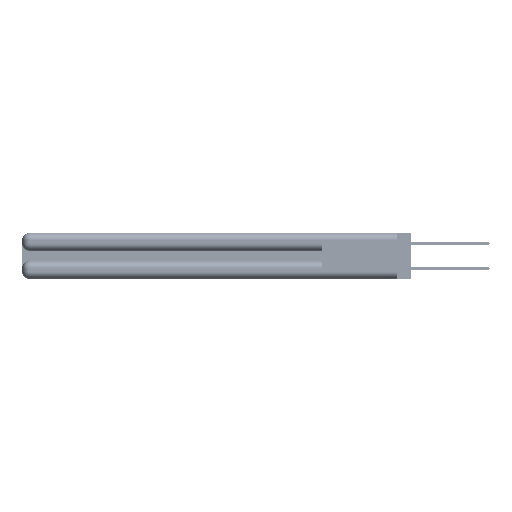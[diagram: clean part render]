
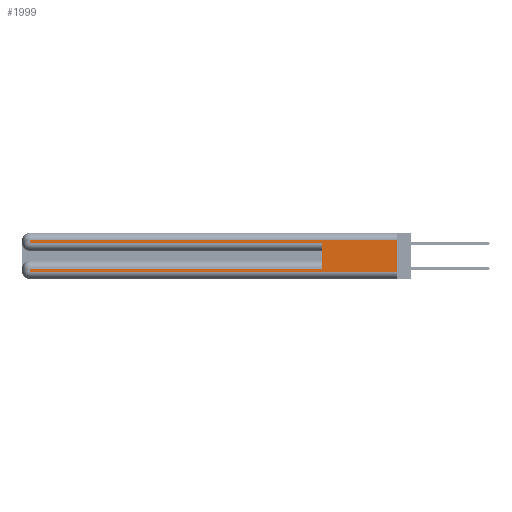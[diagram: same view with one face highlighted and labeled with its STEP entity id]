
A CAD part, left-side view. The second image highlights one B-rep face of the part: STEP entity #1999.
In plain terms, the highlighted planar face has unit normal (-1, 0, 0).
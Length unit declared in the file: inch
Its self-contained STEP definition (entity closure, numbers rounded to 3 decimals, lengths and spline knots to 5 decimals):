
#1750 = FACE_OUTER_BOUND ( 'NONE', #46465, .T. ) ;
#1999 = ADVANCED_FACE ( 'NONE', ( #1750 ), #5914, .F. ) ;
#3607 = ORIENTED_EDGE ( 'NONE', *, *, #37052, .T. ) ;
#3769 = ORIENTED_EDGE ( 'NONE', *, *, #54869, .T. ) ;
#4452 = DIRECTION ( 'NONE',  ( 0., 0., -1. ) ) ;
#4638 = CARTESIAN_POINT ( 'NONE',  ( 0., 2.94, 0.37 ) ) ;
#5604 = LINE ( 'NONE', #4638, #40401 ) ;
#5707 = LINE ( 'NONE', #15758, #15888 ) ;
#5914 = PLANE ( 'NONE',  #20199 ) ;
#6242 = VECTOR ( 'NONE', #30039, 39.37008 ) ;
#8123 = CARTESIAN_POINT ( 'NONE',  ( 0., 0.6, 0.085 ) ) ;
#9010 = DIRECTION ( 'NONE',  ( 0., 0., -1. ) ) ;
#10978 = CARTESIAN_POINT ( 'NONE',  ( 0., 0., 0.085 ) ) ;
#10979 = VECTOR ( 'NONE', #9010, 39.37008 ) ;
#12269 = CARTESIAN_POINT ( 'NONE',  ( 0., 0., 0.31 ) ) ;
#13804 = VECTOR ( 'NONE', #45222, 39.37008 ) ;
#14412 = VERTEX_POINT ( 'NONE', #39367 ) ;
#14622 = DIRECTION ( 'NONE',  ( 0., 0., -1. ) ) ;
#15758 = CARTESIAN_POINT ( 'NONE',  ( 0., 0., 0.37 ) ) ;
#15888 = VECTOR ( 'NONE', #20144, 39.37008 ) ;
#16745 = ORIENTED_EDGE ( 'NONE', *, *, #27738, .F. ) ;
#17822 = LINE ( 'NONE', #25661, #6242 ) ;
#20144 = DIRECTION ( 'NONE',  ( 0., 0., -1. ) ) ;
#20199 = AXIS2_PLACEMENT_3D ( 'NONE', #36408, #40789, #14622 ) ;
#24513 = VERTEX_POINT ( 'NONE', #43925 ) ;
#24615 = ORIENTED_EDGE ( 'NONE', *, *, #28487, .T. ) ;
#24803 = VERTEX_POINT ( 'NONE', #41235 ) ;
#25661 = CARTESIAN_POINT ( 'NONE',  ( 0., 0., 0.06 ) ) ;
#27361 = DIRECTION ( 'NONE',  ( 0., -1., 0. ) ) ;
#27738 = EDGE_CURVE ( 'NONE', #33438, #24513, #5707, .T. ) ;
#28165 = LINE ( 'NONE', #41052, #13804 ) ;
#28487 = EDGE_CURVE ( 'NONE', #36521, #36227, #44465, .T. ) ;
#30039 = DIRECTION ( 'NONE',  ( 0., -1., 0. ) ) ;
#31236 = VERTEX_POINT ( 'NONE', #44261 ) ;
#31534 = VECTOR ( 'NONE', #37148, 39.37008 ) ;
#32031 = VECTOR ( 'NONE', #27361, 39.37008 ) ;
#32733 = CARTESIAN_POINT ( 'NONE',  ( 0., 0.6, 0.145 ) ) ;
#33438 = VERTEX_POINT ( 'NONE', #12269 ) ;
#35183 = CARTESIAN_POINT ( 'NONE',  ( 0., 2.94, 0.37 ) ) ;
#36227 = VERTEX_POINT ( 'NONE', #48456 ) ;
#36408 = CARTESIAN_POINT ( 'NONE',  ( 0., 0., 0.37 ) ) ;
#36521 = VERTEX_POINT ( 'NONE', #41342 ) ;
#37052 = EDGE_CURVE ( 'NONE', #14412, #31236, #43618, .T. ) ;
#37148 = DIRECTION ( 'NONE',  ( 0., 0., 1. ) ) ;
#38247 = LINE ( 'NONE', #10978, #48513 ) ;
#39367 = CARTESIAN_POINT ( 'NONE',  ( 0., 2.94, 0.285 ) ) ;
#40401 = VECTOR ( 'NONE', #4452, 39.37008 ) ;
#40789 = DIRECTION ( 'NONE',  ( 1., 0., 0. ) ) ;
#41052 = CARTESIAN_POINT ( 'NONE',  ( 0., 0., 0.31 ) ) ;
#41235 = CARTESIAN_POINT ( 'NONE',  ( 0., 2.94, 0.31 ) ) ;
#41342 = CARTESIAN_POINT ( 'NONE',  ( 0., 2.94, 0.085 ) ) ;
#41613 = EDGE_CURVE ( 'NONE', #24803, #14412, #5604, .T. ) ;
#43618 = LINE ( 'NONE', #49147, #32031 ) ;
#43657 = ORIENTED_EDGE ( 'NONE', *, *, #52792, .T. ) ;
#43925 = CARTESIAN_POINT ( 'NONE',  ( 0., 0., 0.06 ) ) ;
#44261 = CARTESIAN_POINT ( 'NONE',  ( 0., 0.6, 0.285 ) ) ;
#44465 = LINE ( 'NONE', #35183, #10979 ) ;
#45222 = DIRECTION ( 'NONE',  ( 0., 1., 0. ) ) ;
#46465 = EDGE_LOOP ( 'NONE', ( #16745, #43657, #49325, #3607, #50995, #3769, #24615, #48769 ) ) ;
#47404 = EDGE_CURVE ( 'NONE', #53744, #31236, #54766, .T. ) ;
#47648 = EDGE_CURVE ( 'NONE', #36227, #24513, #17822, .T. ) ;
#48456 = CARTESIAN_POINT ( 'NONE',  ( 0., 2.94, 0.06 ) ) ;
#48513 = VECTOR ( 'NONE', #54754, 39.37008 ) ;
#48769 = ORIENTED_EDGE ( 'NONE', *, *, #47648, .T. ) ;
#49147 = CARTESIAN_POINT ( 'NONE',  ( 0., 0., 0.285 ) ) ;
#49325 = ORIENTED_EDGE ( 'NONE', *, *, #41613, .T. ) ;
#50995 = ORIENTED_EDGE ( 'NONE', *, *, #47404, .F. ) ;
#52792 = EDGE_CURVE ( 'NONE', #33438, #24803, #28165, .T. ) ;
#53744 = VERTEX_POINT ( 'NONE', #8123 ) ;
#54754 = DIRECTION ( 'NONE',  ( 0., 1., 0. ) ) ;
#54766 = LINE ( 'NONE', #32733, #31534 ) ;
#54869 = EDGE_CURVE ( 'NONE', #53744, #36521, #38247, .T. ) ;
